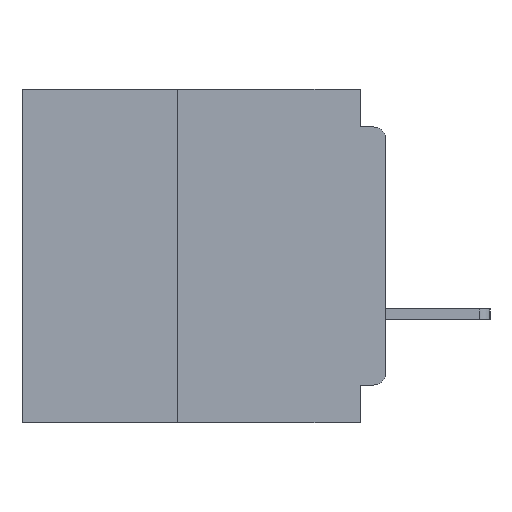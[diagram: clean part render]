
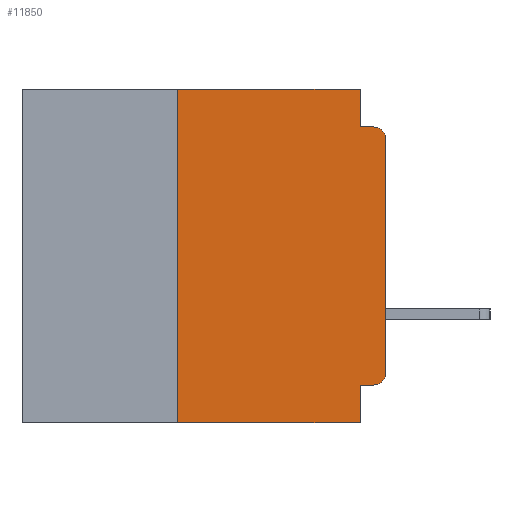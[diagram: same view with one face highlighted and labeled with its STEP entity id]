
A CAD part, left-side view. The second image highlights one B-rep face of the part: STEP entity #11850.
In plain terms, the highlighted planar face has unit normal (-1, 0, 0).
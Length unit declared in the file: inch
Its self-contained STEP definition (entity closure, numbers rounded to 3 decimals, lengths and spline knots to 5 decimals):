
#32 = VECTOR ( 'NONE', #34250, 39.37008 ) ;
#41 = CARTESIAN_POINT ( 'NONE',  ( 0., 0.437, 0. ) ) ;
#383 = DIRECTION ( 'NONE',  ( 0., 0., -1. ) ) ;
#433 = VERTEX_POINT ( 'NONE', #40961 ) ;
#736 = EDGE_CURVE ( 'NONE', #25147, #12345, #43091, .T. ) ;
#1377 = EDGE_LOOP ( 'NONE', ( #28310, #2341, #30145, #18759, #26206, #7082, #47447, #40973, #12693, #5500 ) ) ;
#2341 = ORIENTED_EDGE ( 'NONE', *, *, #9459, .T. ) ;
#3306 = CIRCLE ( 'NONE', #6647, 0.015 ) ;
#4044 = VECTOR ( 'NONE', #44713, 39.37008 ) ;
#4303 = DIRECTION ( 'NONE',  ( 0., -1., 0. ) ) ;
#4925 = VECTOR ( 'NONE', #40083, 39.37008 ) ;
#5267 = LINE ( 'NONE', #18670, #44999 ) ;
#5405 = VECTOR ( 'NONE', #37816, 39.37008 ) ;
#5500 = ORIENTED_EDGE ( 'NONE', *, *, #27744, .T. ) ;
#5739 = VECTOR ( 'NONE', #22894, 39.37008 ) ;
#5985 = EDGE_CURVE ( 'NONE', #11519, #45695, #8101, .T. ) ;
#6647 = AXIS2_PLACEMENT_3D ( 'NONE', #20759, #47626, #24618 ) ;
#7082 = ORIENTED_EDGE ( 'NONE', *, *, #8344, .F. ) ;
#8076 = LINE ( 'NONE', #41057, #37655 ) ;
#8101 = LINE ( 'NONE', #11877, #46647 ) ;
#8344 = EDGE_CURVE ( 'NONE', #22785, #11519, #14270, .T. ) ;
#9459 = EDGE_CURVE ( 'NONE', #12345, #30606, #3306, .T. ) ;
#11501 = LINE ( 'NONE', #14992, #32 ) ;
#11519 = VERTEX_POINT ( 'NONE', #36823 ) ;
#11850 = ADVANCED_FACE ( 'NONE', ( #22416 ), #46502, .F. ) ;
#11877 = CARTESIAN_POINT ( 'NONE',  ( 0., 0.437, 0. ) ) ;
#12345 = VERTEX_POINT ( 'NONE', #37923 ) ;
#12693 = ORIENTED_EDGE ( 'NONE', *, *, #22548, .F. ) ;
#13370 = VERTEX_POINT ( 'NONE', #32748 ) ;
#13739 = CIRCLE ( 'NONE', #37984, 0.015 ) ;
#13945 = LINE ( 'NONE', #47617, #4925 ) ;
#14109 = CARTESIAN_POINT ( 'NONE',  ( 0., 0.015, -0.355 ) ) ;
#14270 = LINE ( 'NONE', #17825, #4044 ) ;
#14992 = CARTESIAN_POINT ( 'NONE',  ( 0., 0., -0.045 ) ) ;
#15200 = AXIS2_PLACEMENT_3D ( 'NONE', #41, #23479, #383 ) ;
#17825 = CARTESIAN_POINT ( 'NONE',  ( 0., 0.25, -0.4 ) ) ;
#18670 = CARTESIAN_POINT ( 'NONE',  ( 0., 0.031, 0. ) ) ;
#18759 = ORIENTED_EDGE ( 'NONE', *, *, #23807, .F. ) ;
#20464 = CARTESIAN_POINT ( 'NONE',  ( 0., 0.015, -0.34 ) ) ;
#20759 = CARTESIAN_POINT ( 'NONE',  ( 0., 0.015, -0.06 ) ) ;
#22416 = FACE_OUTER_BOUND ( 'NONE', #1377, .T. ) ;
#22548 = EDGE_CURVE ( 'NONE', #43185, #433, #24695, .T. ) ;
#22785 = VERTEX_POINT ( 'NONE', #39295 ) ;
#22894 = DIRECTION ( 'NONE',  ( 0., 0., 1. ) ) ;
#23479 = DIRECTION ( 'NONE',  ( 1., 0., 0. ) ) ;
#23807 = EDGE_CURVE ( 'NONE', #45695, #13370, #5267, .T. ) ;
#24315 = DIRECTION ( 'NONE',  ( 0., 0., -1. ) ) ;
#24618 = DIRECTION ( 'NONE',  ( 0., 0., -1. ) ) ;
#24695 = LINE ( 'NONE', #26377, #5405 ) ;
#25147 = VERTEX_POINT ( 'NONE', #26978 ) ;
#26206 = ORIENTED_EDGE ( 'NONE', *, *, #5985, .F. ) ;
#26377 = CARTESIAN_POINT ( 'NONE',  ( 0., 0., -0.355 ) ) ;
#26978 = CARTESIAN_POINT ( 'NONE',  ( 0., 0., -0.34 ) ) ;
#27714 = CARTESIAN_POINT ( 'NONE',  ( 0., 0.015, -0.045 ) ) ;
#27744 = EDGE_CURVE ( 'NONE', #43185, #25147, #13739, .T. ) ;
#28310 = ORIENTED_EDGE ( 'NONE', *, *, #736, .T. ) ;
#28522 = CARTESIAN_POINT ( 'NONE',  ( 0., 0., 0. ) ) ;
#30145 = ORIENTED_EDGE ( 'NONE', *, *, #35126, .F. ) ;
#30606 = VERTEX_POINT ( 'NONE', #27714 ) ;
#32748 = CARTESIAN_POINT ( 'NONE',  ( 0., 0.031, -0.045 ) ) ;
#34034 = DIRECTION ( 'NONE',  ( 0., 0., -1. ) ) ;
#34250 = DIRECTION ( 'NONE',  ( 0., -1., 0. ) ) ;
#35126 = EDGE_CURVE ( 'NONE', #13370, #30606, #11501, .T. ) ;
#36823 = CARTESIAN_POINT ( 'NONE',  ( 0., 0.25, 0. ) ) ;
#37655 = VECTOR ( 'NONE', #48734, 39.37008 ) ;
#37816 = DIRECTION ( 'NONE',  ( 0., 1., 0. ) ) ;
#37923 = CARTESIAN_POINT ( 'NONE',  ( 0., 0., -0.06 ) ) ;
#37984 = AXIS2_PLACEMENT_3D ( 'NONE', #20464, #47327, #24315 ) ;
#38186 = CARTESIAN_POINT ( 'NONE',  ( 0., 0.031, 0. ) ) ;
#39295 = CARTESIAN_POINT ( 'NONE',  ( 0., 0.25, -0.4 ) ) ;
#40083 = DIRECTION ( 'NONE',  ( 0., -1., 0. ) ) ;
#40961 = CARTESIAN_POINT ( 'NONE',  ( 0., 0.031, -0.355 ) ) ;
#40973 = ORIENTED_EDGE ( 'NONE', *, *, #43193, .F. ) ;
#41057 = CARTESIAN_POINT ( 'NONE',  ( 0., 0.031, -0.4 ) ) ;
#41306 = VERTEX_POINT ( 'NONE', #47747 ) ;
#43091 = LINE ( 'NONE', #28522, #5739 ) ;
#43185 = VERTEX_POINT ( 'NONE', #14109 ) ;
#43193 = EDGE_CURVE ( 'NONE', #433, #41306, #8076, .T. ) ;
#44713 = DIRECTION ( 'NONE',  ( 0., 0., 1. ) ) ;
#44999 = VECTOR ( 'NONE', #34034, 39.37008 ) ;
#45695 = VERTEX_POINT ( 'NONE', #38186 ) ;
#46502 = PLANE ( 'NONE',  #15200 ) ;
#46647 = VECTOR ( 'NONE', #4303, 39.37008 ) ;
#47327 = DIRECTION ( 'NONE',  ( -1., 0., 0. ) ) ;
#47447 = ORIENTED_EDGE ( 'NONE', *, *, #49079, .T. ) ;
#47617 = CARTESIAN_POINT ( 'NONE',  ( 0., 0.437, -0.4 ) ) ;
#47626 = DIRECTION ( 'NONE',  ( -1., 0., 0. ) ) ;
#47747 = CARTESIAN_POINT ( 'NONE',  ( 0., 0.031, -0.4 ) ) ;
#48734 = DIRECTION ( 'NONE',  ( 0., 0., -1. ) ) ;
#49079 = EDGE_CURVE ( 'NONE', #22785, #41306, #13945, .T. ) ;
